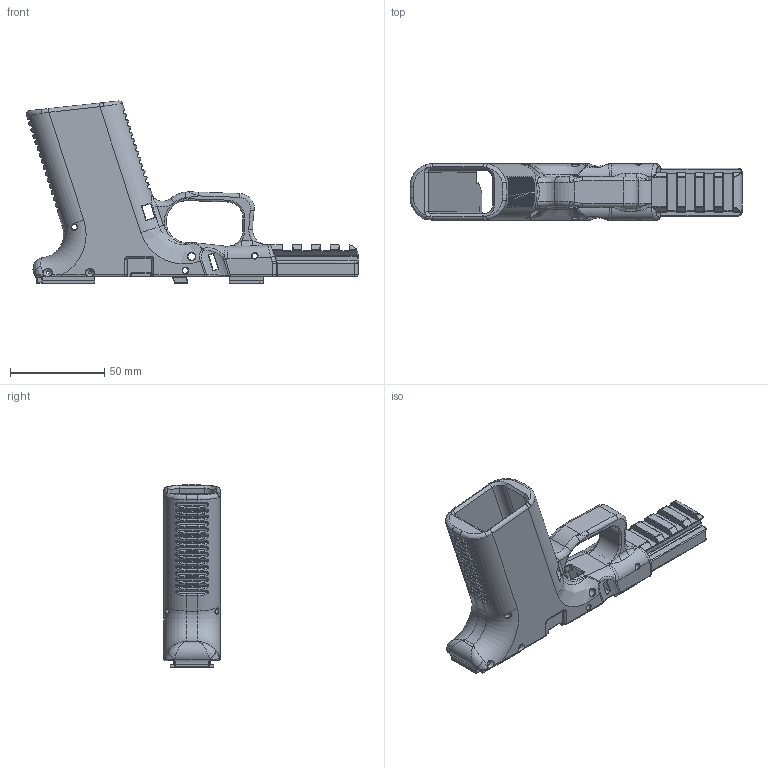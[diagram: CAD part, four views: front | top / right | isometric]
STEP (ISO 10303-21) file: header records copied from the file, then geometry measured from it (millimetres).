
FILE_DESCRIPTION(/* description */ (''),/* implementation_level */ '2;1');
FILE_NAME(/* name */ 'FreeMans Glock 19.step',/* time_stamp */ '2019-09-18T22:13:27-04:00',/* author */ (''),/* organization */ (''),/* preprocessor_version */ 'ST-DEVELOPER v18',/* originating_system */ 'Autodesk Translation Framework v8.6.0.1094',/* authorisation */ '');
FILE_SCHEMA (('AUTOMOTIVE_DESIGN { 1 0 10303 214 3 1 1 }'));
Products named in the file (4): Glock 19 DIY; Front Rail G17 v1; Rear Rail Left; Rear Rail Right
Assembly tree (3 placements, depth 2):
  Glock 19 DIY
    Front Rail G17 v1
    Rear Rail Left
    Rear Rail Right
Bounding box: 176.48 x 30 x 96.84 mm (x, y, z)
Volume: 87272.1 mm3; surface area: 47702.8 mm2
Topology: 4 solids, 4 shells, 1655 faces, 3960 edges, 2225 vertices
Faces by surface type: cylinder 550, bspline 536, plane 332, torus 145, sphere 68, cone 24
Full cylindrical faces by diameter (mm): 1.623 x8, 2.997 x4, 3 x3, 3.962 x2
Entity records: 62548 total; most frequent: CARTESIAN_POINT 26189, ORIENTED_EDGE 7790, DIRECTION 7385, EDGE_CURVE 3895, AXIS2_PLACEMENT_3D 2974, VERTEX_POINT 2231, EDGE_LOOP 1686, FACE_OUTER_BOUND 1655
